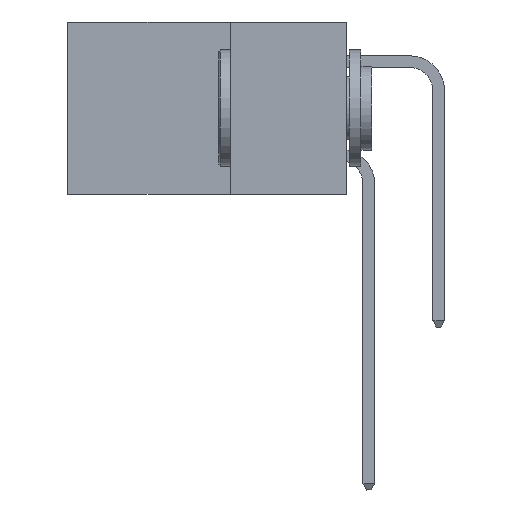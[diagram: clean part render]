
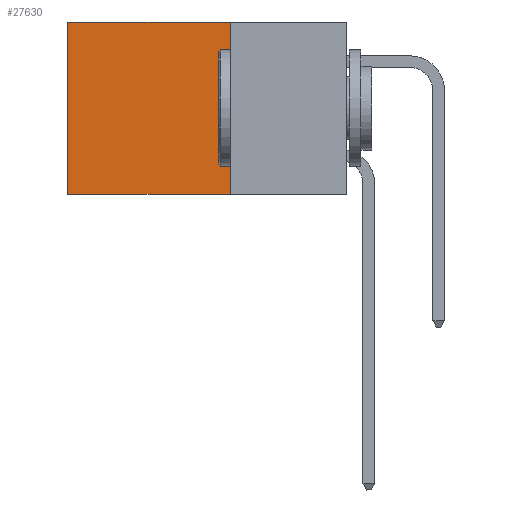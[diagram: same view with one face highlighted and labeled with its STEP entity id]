
A CAD part, left-side view. The second image highlights one B-rep face of the part: STEP entity #27630.
In plain terms, the highlighted planar face has unit normal (-1, 0, 0).
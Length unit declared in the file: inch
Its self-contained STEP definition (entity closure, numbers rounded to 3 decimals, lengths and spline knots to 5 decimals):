
#186 = CARTESIAN_POINT ( 'NONE',  ( 0.2875, 0.6, -0.37 ) ) ;
#312 = CARTESIAN_POINT ( 'NONE',  ( 0.2875, 0.6, 0. ) ) ;
#653 = EDGE_CURVE ( 'NONE', #27438, #2351, #39996, .T. ) ;
#1953 = LINE ( 'NONE', #37836, #15448 ) ;
#2262 = DIRECTION ( 'NONE',  ( 0., 0., -1. ) ) ;
#2351 = VERTEX_POINT ( 'NONE', #186 ) ;
#2564 = LINE ( 'NONE', #11098, #19180 ) ;
#5585 = DIRECTION ( 'NONE',  ( 1., 0., 0. ) ) ;
#6193 = VERTEX_POINT ( 'NONE', #37266 ) ;
#7277 = ORIENTED_EDGE ( 'NONE', *, *, #653, .F. ) ;
#7632 = CARTESIAN_POINT ( 'NONE',  ( 0.2875, 0.25, -0.37 ) ) ;
#11098 = CARTESIAN_POINT ( 'NONE',  ( 0.2875, 0.25, 0. ) ) ;
#12656 = DIRECTION ( 'NONE',  ( 0., 0., -1. ) ) ;
#12939 = CARTESIAN_POINT ( 'NONE',  ( 0.2875, 0.6, 0. ) ) ;
#13840 = EDGE_CURVE ( 'NONE', #38582, #2351, #29014, .T. ) ;
#14864 = EDGE_CURVE ( 'NONE', #6193, #27438, #1953, .T. ) ;
#15448 = VECTOR ( 'NONE', #25011, 39.37008 ) ;
#17329 = EDGE_LOOP ( 'NONE', ( #34454, #7277, #42922, #30045 ) ) ;
#19180 = VECTOR ( 'NONE', #34340, 39.37008 ) ;
#19216 = CARTESIAN_POINT ( 'NONE',  ( 0.2875, 0.25, 0. ) ) ;
#22976 = FACE_OUTER_BOUND ( 'NONE', #17329, .T. ) ;
#24551 = AXIS2_PLACEMENT_3D ( 'NONE', #19216, #5585, #2262 ) ;
#25011 = DIRECTION ( 'NONE',  ( 0., 0., -1. ) ) ;
#26988 = VECTOR ( 'NONE', #41356, 39.37008 ) ;
#27438 = VERTEX_POINT ( 'NONE', #35117 ) ;
#27630 = ADVANCED_FACE ( 'NONE', ( #22976 ), #35555, .F. ) ;
#29014 = LINE ( 'NONE', #12939, #29507 ) ;
#29372 = EDGE_CURVE ( 'NONE', #6193, #38582, #2564, .T. ) ;
#29507 = VECTOR ( 'NONE', #12656, 39.37008 ) ;
#30045 = ORIENTED_EDGE ( 'NONE', *, *, #29372, .T. ) ;
#34340 = DIRECTION ( 'NONE',  ( 0., 1., 0. ) ) ;
#34454 = ORIENTED_EDGE ( 'NONE', *, *, #13840, .T. ) ;
#35117 = CARTESIAN_POINT ( 'NONE',  ( 0.2875, 0.25, -0.37 ) ) ;
#35555 = PLANE ( 'NONE',  #24551 ) ;
#37266 = CARTESIAN_POINT ( 'NONE',  ( 0.2875, 0.25, 0. ) ) ;
#37836 = CARTESIAN_POINT ( 'NONE',  ( 0.2875, 0.25, 0. ) ) ;
#38582 = VERTEX_POINT ( 'NONE', #312 ) ;
#39996 = LINE ( 'NONE', #7632, #26988 ) ;
#41356 = DIRECTION ( 'NONE',  ( 0., 1., 0. ) ) ;
#42922 = ORIENTED_EDGE ( 'NONE', *, *, #14864, .F. ) ;
